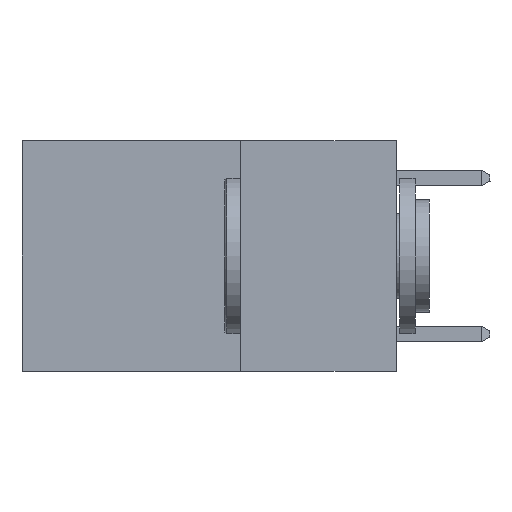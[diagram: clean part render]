
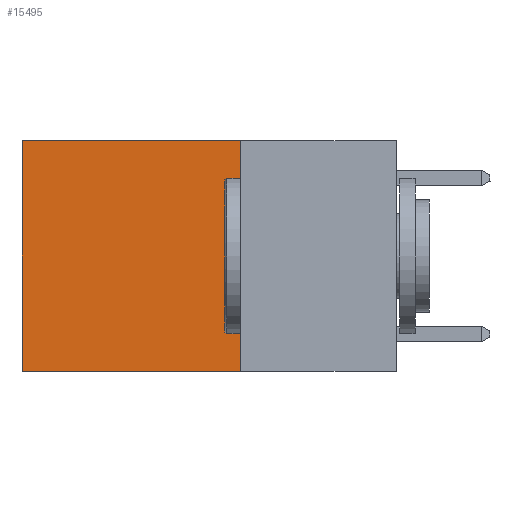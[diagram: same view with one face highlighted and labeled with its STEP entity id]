
A CAD part, left-side view. The second image highlights one B-rep face of the part: STEP entity #15495.
In plain terms, the highlighted planar face has unit normal (-1, 0, 0).
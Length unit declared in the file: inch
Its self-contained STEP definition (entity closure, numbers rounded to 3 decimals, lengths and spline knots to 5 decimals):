
#1762 = CARTESIAN_POINT ( 'NONE',  ( 0.2625, 0.6, 0. ) ) ;
#1813 = FACE_OUTER_BOUND ( 'NONE', #7995, .T. ) ;
#2229 = DIRECTION ( 'NONE',  ( 0., 0., -1. ) ) ;
#2940 = ORIENTED_EDGE ( 'NONE', *, *, #10119, .F. ) ;
#3258 = CARTESIAN_POINT ( 'NONE',  ( 0.2625, 0.6, 0. ) ) ;
#3778 = CARTESIAN_POINT ( 'NONE',  ( 0.2625, 0.25, 0. ) ) ;
#4578 = EDGE_CURVE ( 'NONE', #12034, #7513, #9092, .T. ) ;
#6436 = VECTOR ( 'NONE', #14232, 39.37008 ) ;
#6890 = CARTESIAN_POINT ( 'NONE',  ( 0.2625, 0.25, -0.37 ) ) ;
#7107 = CARTESIAN_POINT ( 'NONE',  ( 0.2625, 0.25, 0. ) ) ;
#7513 = VERTEX_POINT ( 'NONE', #9805 ) ;
#7720 = LINE ( 'NONE', #3778, #14101 ) ;
#7897 = ORIENTED_EDGE ( 'NONE', *, *, #13039, .F. ) ;
#7995 = EDGE_LOOP ( 'NONE', ( #13810, #7897, #2940, #8012 ) ) ;
#8012 = ORIENTED_EDGE ( 'NONE', *, *, #15843, .T. ) ;
#8378 = DIRECTION ( 'NONE',  ( 0., 0., -1. ) ) ;
#8521 = CARTESIAN_POINT ( 'NONE',  ( 0.2625, 0.25, 0. ) ) ;
#8716 = CARTESIAN_POINT ( 'NONE',  ( 0.2625, 0.25, 0. ) ) ;
#8737 = AXIS2_PLACEMENT_3D ( 'NONE', #7107, #15943, #8378 ) ;
#8816 = VERTEX_POINT ( 'NONE', #8521 ) ;
#9092 = LINE ( 'NONE', #1762, #15431 ) ;
#9266 = VECTOR ( 'NONE', #2229, 39.37008 ) ;
#9528 = DIRECTION ( 'NONE',  ( 0., 0., -1. ) ) ;
#9805 = CARTESIAN_POINT ( 'NONE',  ( 0.2625, 0.6, -0.37 ) ) ;
#10119 = EDGE_CURVE ( 'NONE', #8816, #13204, #12667, .T. ) ;
#10213 = LINE ( 'NONE', #14173, #6436 ) ;
#11476 = DIRECTION ( 'NONE',  ( 0., 1., 0. ) ) ;
#12034 = VERTEX_POINT ( 'NONE', #3258 ) ;
#12667 = LINE ( 'NONE', #8716, #9266 ) ;
#13039 = EDGE_CURVE ( 'NONE', #13204, #7513, #10213, .T. ) ;
#13204 = VERTEX_POINT ( 'NONE', #6890 ) ;
#13426 = PLANE ( 'NONE',  #8737 ) ;
#13810 = ORIENTED_EDGE ( 'NONE', *, *, #4578, .T. ) ;
#14101 = VECTOR ( 'NONE', #11476, 39.37008 ) ;
#14173 = CARTESIAN_POINT ( 'NONE',  ( 0.2625, 0.25, -0.37 ) ) ;
#14232 = DIRECTION ( 'NONE',  ( 0., 1., 0. ) ) ;
#15431 = VECTOR ( 'NONE', #9528, 39.37008 ) ;
#15495 = ADVANCED_FACE ( 'NONE', ( #1813 ), #13426, .F. ) ;
#15843 = EDGE_CURVE ( 'NONE', #8816, #12034, #7720, .T. ) ;
#15943 = DIRECTION ( 'NONE',  ( 1., 0., 0. ) ) ;
